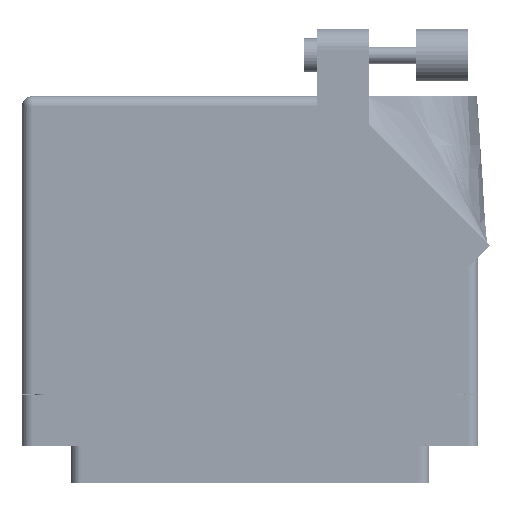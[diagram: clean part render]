
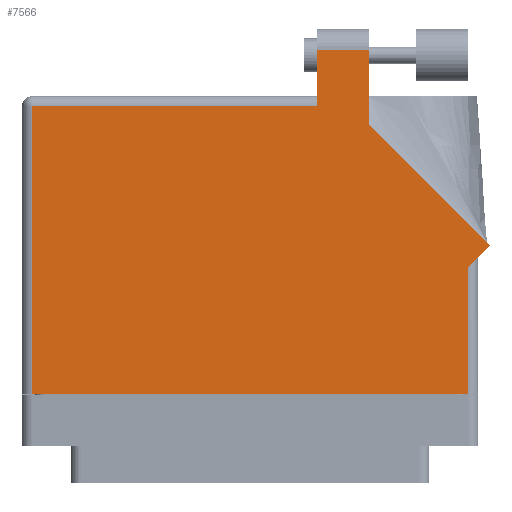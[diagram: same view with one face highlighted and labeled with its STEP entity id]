
A CAD part, front view. The second image highlights one B-rep face of the part: STEP entity #7566.
In plain terms, the highlighted face is planar.
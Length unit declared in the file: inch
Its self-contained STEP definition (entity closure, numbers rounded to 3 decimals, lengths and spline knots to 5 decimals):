
#1377 = ORIENTED_EDGE ( 'NONE', *, *, #44730, .T. ) ;
#2114 = CARTESIAN_POINT ( 'NONE',  ( 1.297, -0.1, 0.617 ) ) ;
#2957 = VECTOR ( 'NONE', #59930, 39.37008 ) ;
#4717 = DIRECTION ( 'NONE',  ( -1., 0., 0. ) ) ;
#5224 = LINE ( 'NONE', #68635, #50228 ) ;
#5968 = VECTOR ( 'NONE', #50510, 39.37008 ) ;
#7566 = ADVANCED_FACE ( 'NONE', ( #20459 ), #51788, .F. ) ;
#7835 = ORIENTED_EDGE ( 'NONE', *, *, #38553, .T. ) ;
#8780 = CARTESIAN_POINT ( 'NONE',  ( 0.706, 1.50942, 0.617 ) ) ;
#15005 = CARTESIAN_POINT ( 'NONE',  ( 1.297, 0.653, 0.617 ) ) ;
#18368 = VECTOR ( 'NONE', #34934, 39.37008 ) ;
#20342 = DIRECTION ( 'NONE',  ( -1., 0., 0. ) ) ;
#20459 = FACE_OUTER_BOUND ( 'NONE', #63116, .T. ) ;
#21299 = DIRECTION ( 'NONE',  ( -0.707, 0.707, 0. ) ) ;
#23846 = CARTESIAN_POINT ( 'NONE',  ( 0.706, 1.95, 0.617 ) ) ;
#24174 = EDGE_CURVE ( 'NONE', #65542, #68042, #27608, .T. ) ;
#25967 = LINE ( 'NONE', #26538, #2957 ) ;
#26047 = EDGE_CURVE ( 'NONE', #68042, #26184, #58691, .T. ) ;
#26184 = VERTEX_POINT ( 'NONE', #2114 ) ;
#26482 = VECTOR ( 'NONE', #47220, 39.37008 ) ;
#26538 = CARTESIAN_POINT ( 'NONE',  ( 0.706, 1.50942, 0.617 ) ) ;
#27608 = LINE ( 'NONE', #35408, #18368 ) ;
#27665 = LINE ( 'NONE', #31056, #55664 ) ;
#30807 = EDGE_CURVE ( 'NONE', #52480, #35423, #52669, .T. ) ;
#31056 = CARTESIAN_POINT ( 'NONE',  ( 0.399, 1.95, 0.617 ) ) ;
#31068 = CARTESIAN_POINT ( 'NONE',  ( 0.399, 1.613, 0.617 ) ) ;
#33027 = DIRECTION ( 'NONE',  ( 0., 1., 0. ) ) ;
#33609 = EDGE_CURVE ( 'NONE', #46125, #65542, #33770, .T. ) ;
#33770 = LINE ( 'NONE', #53656, #61709 ) ;
#34934 = DIRECTION ( 'NONE',  ( 0., -1., 0. ) ) ;
#35298 = ORIENTED_EDGE ( 'NONE', *, *, #33609, .T. ) ;
#35386 = VERTEX_POINT ( 'NONE', #8780 ) ;
#35408 = CARTESIAN_POINT ( 'NONE',  ( -1.297, -0.1, 0.617 ) ) ;
#35423 = VERTEX_POINT ( 'NONE', #62402 ) ;
#38553 = EDGE_CURVE ( 'NONE', #35386, #59114, #25967, .T. ) ;
#40700 = AXIS2_PLACEMENT_3D ( 'NONE', #46829, #52264, #20342 ) ;
#43434 = DIRECTION ( 'NONE',  ( -1., 0., 0. ) ) ;
#43555 = EDGE_CURVE ( 'NONE', #26184, #52480, #63433, .T. ) ;
#43696 = CARTESIAN_POINT ( 'NONE',  ( 1.42971, 0.78571, 0.617 ) ) ;
#44730 = EDGE_CURVE ( 'NONE', #59114, #64918, #27665, .T. ) ;
#46125 = VERTEX_POINT ( 'NONE', #31068 ) ;
#46829 = CARTESIAN_POINT ( 'NONE',  ( -1.359, 1.675, 0.617 ) ) ;
#47075 = DIRECTION ( 'NONE',  ( 0., -1., 0. ) ) ;
#47220 = DIRECTION ( 'NONE',  ( 1., 0., 0. ) ) ;
#48228 = ORIENTED_EDGE ( 'NONE', *, *, #30807, .T. ) ;
#48439 = CARTESIAN_POINT ( 'NONE',  ( 1.297, 0.715, 0.617 ) ) ;
#49183 = CARTESIAN_POINT ( 'NONE',  ( -1.297, -0.1, 0.617 ) ) ;
#50228 = VECTOR ( 'NONE', #47075, 39.37008 ) ;
#50442 = ORIENTED_EDGE ( 'NONE', *, *, #55888, .T. ) ;
#50510 = DIRECTION ( 'NONE',  ( 0.707, 0.707, 0. ) ) ;
#51788 = PLANE ( 'NONE',  #40700 ) ;
#52264 = DIRECTION ( 'NONE',  ( 0., 0., -1. ) ) ;
#52480 = VERTEX_POINT ( 'NONE', #15005 ) ;
#52669 = LINE ( 'NONE', #66619, #5968 ) ;
#53219 = ORIENTED_EDGE ( 'NONE', *, *, #24174, .T. ) ;
#53656 = CARTESIAN_POINT ( 'NONE',  ( -1.359, 1.613, 0.617 ) ) ;
#55664 = VECTOR ( 'NONE', #4717, 39.37008 ) ;
#55888 = EDGE_CURVE ( 'NONE', #64918, #46125, #5224, .T. ) ;
#56367 = ORIENTED_EDGE ( 'NONE', *, *, #26047, .T. ) ;
#58423 = ORIENTED_EDGE ( 'NONE', *, *, #43555, .T. ) ;
#58691 = LINE ( 'NONE', #64052, #26482 ) ;
#59114 = VERTEX_POINT ( 'NONE', #23846 ) ;
#59135 = LINE ( 'NONE', #43696, #67621 ) ;
#59930 = DIRECTION ( 'NONE',  ( 0., 1., 0. ) ) ;
#60173 = ORIENTED_EDGE ( 'NONE', *, *, #66226, .T. ) ;
#61709 = VECTOR ( 'NONE', #43434, 39.37008 ) ;
#62402 = CARTESIAN_POINT ( 'NONE',  ( 1.42971, 0.78571, 0.617 ) ) ;
#63116 = EDGE_LOOP ( 'NONE', ( #7835, #1377, #50442, #35298, #53219, #56367, #58423, #48228, #60173 ) ) ;
#63433 = LINE ( 'NONE', #48439, #64324 ) ;
#64052 = CARTESIAN_POINT ( 'NONE',  ( -1.359, -0.1, 0.617 ) ) ;
#64324 = VECTOR ( 'NONE', #33027, 39.37008 ) ;
#64385 = CARTESIAN_POINT ( 'NONE',  ( 0.399, 1.95, 0.617 ) ) ;
#64918 = VERTEX_POINT ( 'NONE', #64385 ) ;
#65542 = VERTEX_POINT ( 'NONE', #66182 ) ;
#66182 = CARTESIAN_POINT ( 'NONE',  ( -1.297, 1.613, 0.617 ) ) ;
#66226 = EDGE_CURVE ( 'NONE', #35423, #35386, #59135, .T. ) ;
#66619 = CARTESIAN_POINT ( 'NONE',  ( 1.359, 0.715, 0.617 ) ) ;
#67621 = VECTOR ( 'NONE', #21299, 39.37008 ) ;
#68042 = VERTEX_POINT ( 'NONE', #49183 ) ;
#68635 = CARTESIAN_POINT ( 'NONE',  ( 0.399, 1.675, 0.617 ) ) ;
